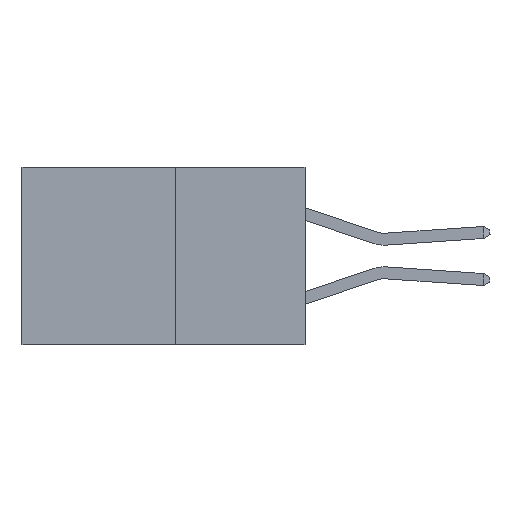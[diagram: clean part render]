
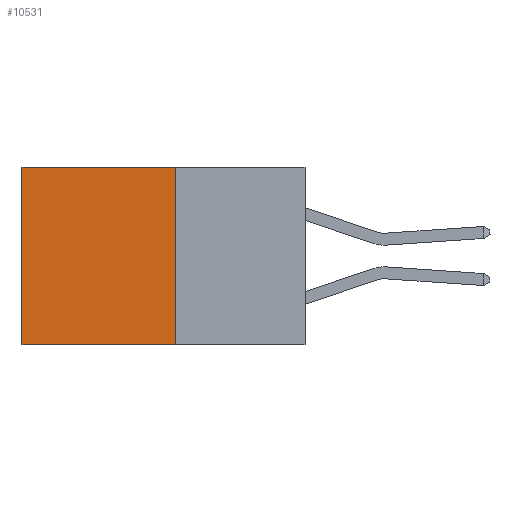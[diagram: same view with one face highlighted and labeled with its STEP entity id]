
A CAD part, left-side view. The second image highlights one B-rep face of the part: STEP entity #10531.
In plain terms, the highlighted planar face has unit normal (-1, 0, 0).
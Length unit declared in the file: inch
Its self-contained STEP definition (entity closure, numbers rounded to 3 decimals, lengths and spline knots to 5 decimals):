
#1108 = VECTOR ( 'NONE', #2747, 39.37008 ) ;
#1114 = ORIENTED_EDGE ( 'NONE', *, *, #9127, .F. ) ;
#1750 = CARTESIAN_POINT ( 'NONE',  ( 0.277, 0.27, -0.37 ) ) ;
#1871 = DIRECTION ( 'NONE',  ( 0., 0., -1. ) ) ;
#2320 = VERTEX_POINT ( 'NONE', #12347 ) ;
#2358 = VECTOR ( 'NONE', #1871, 39.37008 ) ;
#2462 = CARTESIAN_POINT ( 'NONE',  ( 0.277, 0.27, -0.37 ) ) ;
#2691 = EDGE_CURVE ( 'NONE', #9645, #3654, #7613, .T. ) ;
#2699 = LINE ( 'NONE', #2462, #2358 ) ;
#2747 = DIRECTION ( 'NONE',  ( 0., 0., -1. ) ) ;
#2882 = DIRECTION ( 'NONE',  ( 0., 1., 0. ) ) ;
#3391 = ORIENTED_EDGE ( 'NONE', *, *, #12813, .T. ) ;
#3654 = VERTEX_POINT ( 'NONE', #6061 ) ;
#3835 = DIRECTION ( 'NONE',  ( 0., 1., 0. ) ) ;
#4069 = LINE ( 'NONE', #4922, #1108 ) ;
#4100 = CARTESIAN_POINT ( 'NONE',  ( 0.277, 0.27, 0. ) ) ;
#4762 = VECTOR ( 'NONE', #3835, 39.37008 ) ;
#4922 = CARTESIAN_POINT ( 'NONE',  ( 0.277, 0.59, -0.37 ) ) ;
#5466 = DIRECTION ( 'NONE',  ( 0., 0., -1. ) ) ;
#5746 = AXIS2_PLACEMENT_3D ( 'NONE', #9635, #11762, #5466 ) ;
#6061 = CARTESIAN_POINT ( 'NONE',  ( 0.277, 0.59, 0. ) ) ;
#7255 = EDGE_LOOP ( 'NONE', ( #3391, #1114, #9708, #7278 ) ) ;
#7278 = ORIENTED_EDGE ( 'NONE', *, *, #2691, .T. ) ;
#7613 = LINE ( 'NONE', #4100, #4762 ) ;
#7625 = EDGE_CURVE ( 'NONE', #9645, #2320, #2699, .T. ) ;
#8367 = CARTESIAN_POINT ( 'NONE',  ( 0.277, 0.59, -0.37 ) ) ;
#9127 = EDGE_CURVE ( 'NONE', #2320, #11652, #12419, .T. ) ;
#9635 = CARTESIAN_POINT ( 'NONE',  ( 0.277, 0.27, -0.37 ) ) ;
#9645 = VERTEX_POINT ( 'NONE', #10262 ) ;
#9708 = ORIENTED_EDGE ( 'NONE', *, *, #7625, .F. ) ;
#10262 = CARTESIAN_POINT ( 'NONE',  ( 0.277, 0.27, 0. ) ) ;
#10531 = ADVANCED_FACE ( 'NONE', ( #13127 ), #10689, .F. ) ;
#10689 = PLANE ( 'NONE',  #5746 ) ;
#11652 = VERTEX_POINT ( 'NONE', #8367 ) ;
#11762 = DIRECTION ( 'NONE',  ( 1., 0., 0. ) ) ;
#12086 = VECTOR ( 'NONE', #2882, 39.37008 ) ;
#12347 = CARTESIAN_POINT ( 'NONE',  ( 0.277, 0.27, -0.37 ) ) ;
#12419 = LINE ( 'NONE', #1750, #12086 ) ;
#12813 = EDGE_CURVE ( 'NONE', #3654, #11652, #4069, .T. ) ;
#13127 = FACE_OUTER_BOUND ( 'NONE', #7255, .T. ) ;
